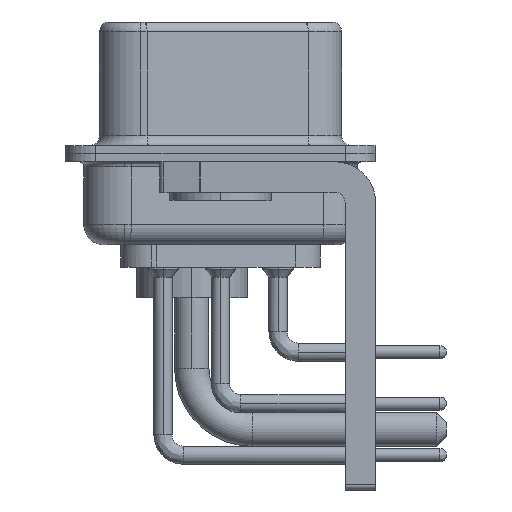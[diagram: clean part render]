
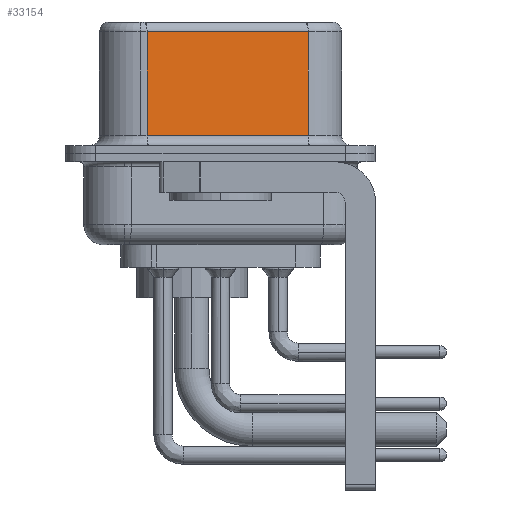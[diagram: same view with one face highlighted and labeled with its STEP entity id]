
A CAD part, left-side view. The second image highlights one B-rep face of the part: STEP entity #33154.
In plain terms, the highlighted planar face has unit normal (-0.985, -0.174, 0).
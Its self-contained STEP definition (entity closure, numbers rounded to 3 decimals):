
#48 = ORIENTED_EDGE ( 'NONE', *, *, #31091, .T. ) ;
#971 = CARTESIAN_POINT ( 'NONE',  ( 5.132, -4.322, 0.9 ) ) ;
#2816 = DIRECTION ( 'NONE',  ( -0.174, 0.985, 0. ) ) ;
#3233 = DIRECTION ( 'NONE',  ( -0.174, 0.985, 0. ) ) ;
#3821 = EDGE_LOOP ( 'NONE', ( #29775, #26069, #27949, #48 ) ) ;
#3990 = EDGE_CURVE ( 'NONE', #34706, #34633, #17456, .T. ) ;
#5631 = CARTESIAN_POINT ( 'NONE',  ( 3.73, 3.628, 6.52 ) ) ;
#5962 = VERTEX_POINT ( 'NONE', #28581 ) ;
#6981 = DIRECTION ( 'NONE',  ( 0.174, -0.985, 0. ) ) ;
#10952 = DIRECTION ( 'NONE',  ( 0., 0., -1. ) ) ;
#11290 = VECTOR ( 'NONE', #6981, 1000. ) ;
#11466 = CARTESIAN_POINT ( 'NONE',  ( 5.132, -4.322, 6.52 ) ) ;
#11639 = DIRECTION ( 'NONE',  ( 0., 0., -1. ) ) ;
#14671 = CARTESIAN_POINT ( 'NONE',  ( 5.132, -4.322, 6.02 ) ) ;
#16220 = CARTESIAN_POINT ( 'NONE',  ( 3.73, 3.628, 0.9 ) ) ;
#16877 = PLANE ( 'NONE',  #28047 ) ;
#17456 = LINE ( 'NONE', #14671, #23623 ) ;
#19310 = FACE_OUTER_BOUND ( 'NONE', #3821, .T. ) ;
#19689 = DIRECTION ( 'NONE',  ( 0.985, 0.174, 0. ) ) ;
#23232 = LINE ( 'NONE', #5631, #29931 ) ;
#23435 = CARTESIAN_POINT ( 'NONE',  ( 5.132, -4.322, 6.02 ) ) ;
#23623 = VECTOR ( 'NONE', #3233, 1000. ) ;
#24106 = CARTESIAN_POINT ( 'NONE',  ( 5.132, -4.322, 6.52 ) ) ;
#25506 = CARTESIAN_POINT ( 'NONE',  ( 3.73, 3.628, 6.02 ) ) ;
#26069 = ORIENTED_EDGE ( 'NONE', *, *, #3990, .T. ) ;
#26621 = LINE ( 'NONE', #971, #11290 ) ;
#27949 = ORIENTED_EDGE ( 'NONE', *, *, #28089, .T. ) ;
#28047 = AXIS2_PLACEMENT_3D ( 'NONE', #11466, #19689, #2816 ) ;
#28089 = EDGE_CURVE ( 'NONE', #34633, #32087, #23232, .T. ) ;
#28581 = CARTESIAN_POINT ( 'NONE',  ( 5.132, -4.322, 0.9 ) ) ;
#29775 = ORIENTED_EDGE ( 'NONE', *, *, #33896, .F. ) ;
#29931 = VECTOR ( 'NONE', #11639, 1000. ) ;
#31091 = EDGE_CURVE ( 'NONE', #32087, #5962, #26621, .T. ) ;
#32087 = VERTEX_POINT ( 'NONE', #16220 ) ;
#33154 = ADVANCED_FACE ( 'NONE', ( #19310 ), #16877, .F. ) ;
#33896 = EDGE_CURVE ( 'NONE', #34706, #5962, #35331, .T. ) ;
#34633 = VERTEX_POINT ( 'NONE', #25506 ) ;
#34663 = VECTOR ( 'NONE', #10952, 1000. ) ;
#34706 = VERTEX_POINT ( 'NONE', #23435 ) ;
#35331 = LINE ( 'NONE', #24106, #34663 ) ;
